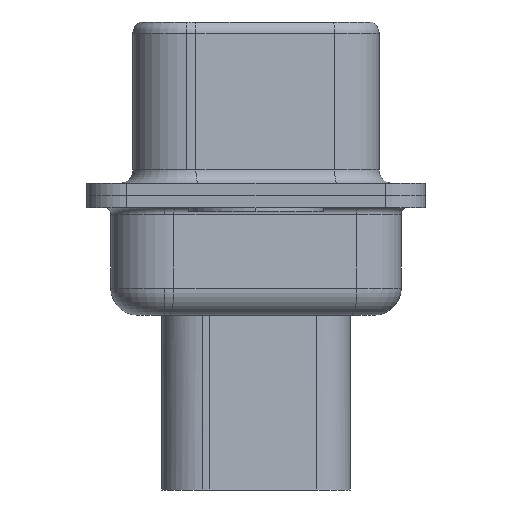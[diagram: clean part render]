
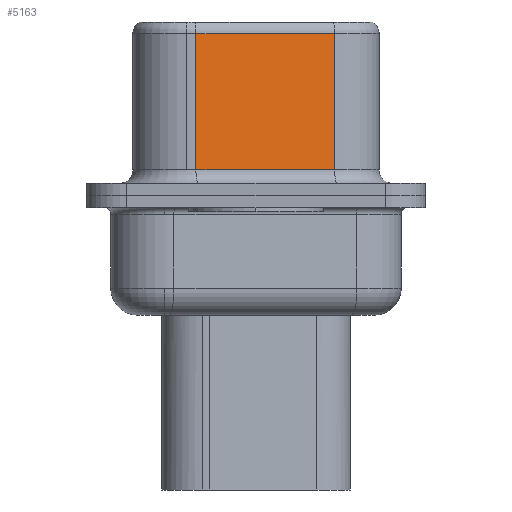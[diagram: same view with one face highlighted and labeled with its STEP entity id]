
A CAD part, left-side view. The second image highlights one B-rep face of the part: STEP entity #5163.
In plain terms, the highlighted planar face has unit normal (-0.985, -0.174, 0).
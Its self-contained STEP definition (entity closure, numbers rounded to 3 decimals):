
#824 = CARTESIAN_POINT ( 'NONE',  ( 3.665, 2.233, 0.95 ) ) ;
#999 = DIRECTION ( 'NONE',  ( 0., 0., -1. ) ) ;
#1052 = CARTESIAN_POINT ( 'NONE',  ( 3.665, 2.233, 6.52 ) ) ;
#1064 = DIRECTION ( 'NONE',  ( -0.174, 0.985, 0. ) ) ;
#1116 = VERTEX_POINT ( 'NONE', #5046 ) ;
#1229 = VECTOR ( 'NONE', #5502, 1000. ) ;
#1296 = LINE ( 'NONE', #6055, #7489 ) ;
#2175 = VERTEX_POINT ( 'NONE', #824 ) ;
#3075 = VECTOR ( 'NONE', #999, 1000. ) ;
#3114 = EDGE_CURVE ( 'NONE', #5364, #6559, #8076, .T. ) ;
#3542 = EDGE_LOOP ( 'NONE', ( #4427, #8977, #8914, #9825 ) ) ;
#4365 = VECTOR ( 'NONE', #5781, 1000. ) ;
#4427 = ORIENTED_EDGE ( 'NONE', *, *, #3114, .F. ) ;
#5046 = CARTESIAN_POINT ( 'NONE',  ( 3.665, 2.233, 6.02 ) ) ;
#5163 = ADVANCED_FACE ( 'NONE', ( #8776 ), #6666, .F. ) ;
#5349 = CARTESIAN_POINT ( 'NONE',  ( 4.575, -2.927, 6.02 ) ) ;
#5364 = VERTEX_POINT ( 'NONE', #5349 ) ;
#5502 = DIRECTION ( 'NONE',  ( -0.174, 0.985, 0. ) ) ;
#5634 = EDGE_CURVE ( 'NONE', #1116, #2175, #8918, .T. ) ;
#5718 = CARTESIAN_POINT ( 'NONE',  ( 4.575, -2.927, 6.52 ) ) ;
#5781 = DIRECTION ( 'NONE',  ( 0., 0., -1. ) ) ;
#6055 = CARTESIAN_POINT ( 'NONE',  ( 4.575, -2.927, 0.95 ) ) ;
#6370 = AXIS2_PLACEMENT_3D ( 'NONE', #8242, #6520, #1064 ) ;
#6520 = DIRECTION ( 'NONE',  ( 0.985, 0.174, 0. ) ) ;
#6559 = VERTEX_POINT ( 'NONE', #9110 ) ;
#6666 = PLANE ( 'NONE',  #6370 ) ;
#6772 = EDGE_CURVE ( 'NONE', #5364, #1116, #9591, .T. ) ;
#7489 = VECTOR ( 'NONE', #8514, 1000. ) ;
#7822 = EDGE_CURVE ( 'NONE', #2175, #6559, #1296, .T. ) ;
#7914 = CARTESIAN_POINT ( 'NONE',  ( 4.575, -2.927, 6.02 ) ) ;
#8076 = LINE ( 'NONE', #5718, #3075 ) ;
#8242 = CARTESIAN_POINT ( 'NONE',  ( 4.575, -2.927, 6.52 ) ) ;
#8514 = DIRECTION ( 'NONE',  ( 0.174, -0.985, 0. ) ) ;
#8776 = FACE_OUTER_BOUND ( 'NONE', #3542, .T. ) ;
#8914 = ORIENTED_EDGE ( 'NONE', *, *, #5634, .T. ) ;
#8918 = LINE ( 'NONE', #1052, #4365 ) ;
#8977 = ORIENTED_EDGE ( 'NONE', *, *, #6772, .T. ) ;
#9110 = CARTESIAN_POINT ( 'NONE',  ( 4.575, -2.927, 0.95 ) ) ;
#9591 = LINE ( 'NONE', #7914, #1229 ) ;
#9825 = ORIENTED_EDGE ( 'NONE', *, *, #7822, .T. ) ;
